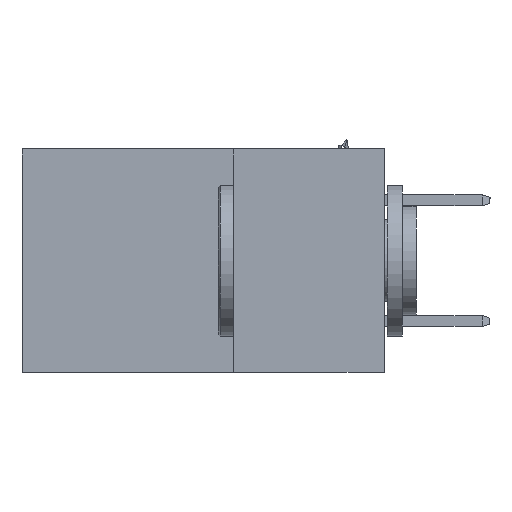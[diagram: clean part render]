
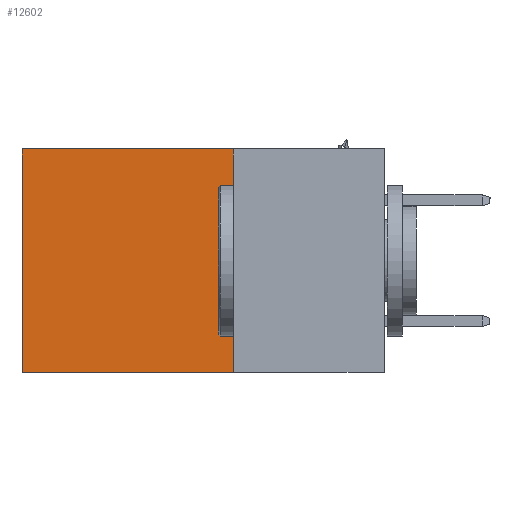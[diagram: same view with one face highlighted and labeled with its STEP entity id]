
A CAD part, left-side view. The second image highlights one B-rep face of the part: STEP entity #12602.
In plain terms, the highlighted planar face has unit normal (-1, 0, 0).
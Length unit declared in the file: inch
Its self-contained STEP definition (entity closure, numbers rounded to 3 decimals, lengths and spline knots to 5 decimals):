
#1570 = VECTOR ( 'NONE', #19578, 39.37008 ) ;
#1907 = PLANE ( 'NONE',  #22629 ) ;
#2302 = EDGE_CURVE ( 'NONE', #12476, #27409, #4677, .T. ) ;
#3493 = VERTEX_POINT ( 'NONE', #11119 ) ;
#4191 = CARTESIAN_POINT ( 'NONE',  ( 0.2615, 0.25, -0.37 ) ) ;
#4677 = LINE ( 'NONE', #11120, #13510 ) ;
#4887 = CARTESIAN_POINT ( 'NONE',  ( 0.2615, 0.25, -0.37 ) ) ;
#6213 = CARTESIAN_POINT ( 'NONE',  ( 0.2615, 0.6, -0.37 ) ) ;
#6499 = DIRECTION ( 'NONE',  ( 0., 0., -1. ) ) ;
#7329 = VERTEX_POINT ( 'NONE', #17697 ) ;
#7423 = DIRECTION ( 'NONE',  ( 0., 1., 0. ) ) ;
#11119 = CARTESIAN_POINT ( 'NONE',  ( 0.2615, 0.6, 0. ) ) ;
#11120 = CARTESIAN_POINT ( 'NONE',  ( 0.2615, 0.25, -0.37 ) ) ;
#12220 = ORIENTED_EDGE ( 'NONE', *, *, #25107, .T. ) ;
#12476 = VERTEX_POINT ( 'NONE', #16535 ) ;
#12602 = ADVANCED_FACE ( 'NONE', ( #15228 ), #1907, .F. ) ;
#13127 = CARTESIAN_POINT ( 'NONE',  ( 0.2615, 0.25, 0. ) ) ;
#13510 = VECTOR ( 'NONE', #26318, 39.37008 ) ;
#14364 = ORIENTED_EDGE ( 'NONE', *, *, #21922, .F. ) ;
#14980 = LINE ( 'NONE', #13127, #1570 ) ;
#15228 = FACE_OUTER_BOUND ( 'NONE', #21390, .T. ) ;
#15764 = CARTESIAN_POINT ( 'NONE',  ( 0.2615, 0.25, -0.37 ) ) ;
#16535 = CARTESIAN_POINT ( 'NONE',  ( 0.2615, 0.25, 0. ) ) ;
#16906 = EDGE_CURVE ( 'NONE', #3493, #7329, #23976, .T. ) ;
#17697 = CARTESIAN_POINT ( 'NONE',  ( 0.2615, 0.6, -0.37 ) ) ;
#19400 = DIRECTION ( 'NONE',  ( 0., 0., -1. ) ) ;
#19578 = DIRECTION ( 'NONE',  ( 0., 1., 0. ) ) ;
#20995 = ORIENTED_EDGE ( 'NONE', *, *, #2302, .F. ) ;
#21390 = EDGE_LOOP ( 'NONE', ( #23248, #14364, #20995, #12220 ) ) ;
#21535 = DIRECTION ( 'NONE',  ( 1., 0., 0. ) ) ;
#21922 = EDGE_CURVE ( 'NONE', #27409, #7329, #24347, .T. ) ;
#22500 = VECTOR ( 'NONE', #7423, 39.37008 ) ;
#22629 = AXIS2_PLACEMENT_3D ( 'NONE', #4191, #21535, #19400 ) ;
#23248 = ORIENTED_EDGE ( 'NONE', *, *, #16906, .T. ) ;
#23627 = VECTOR ( 'NONE', #6499, 39.37008 ) ;
#23976 = LINE ( 'NONE', #6213, #23627 ) ;
#24347 = LINE ( 'NONE', #15764, #22500 ) ;
#25107 = EDGE_CURVE ( 'NONE', #12476, #3493, #14980, .T. ) ;
#26318 = DIRECTION ( 'NONE',  ( 0., 0., -1. ) ) ;
#27409 = VERTEX_POINT ( 'NONE', #4887 ) ;
